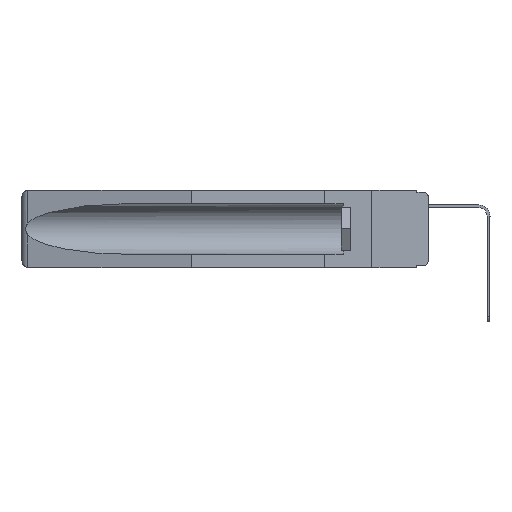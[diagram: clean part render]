
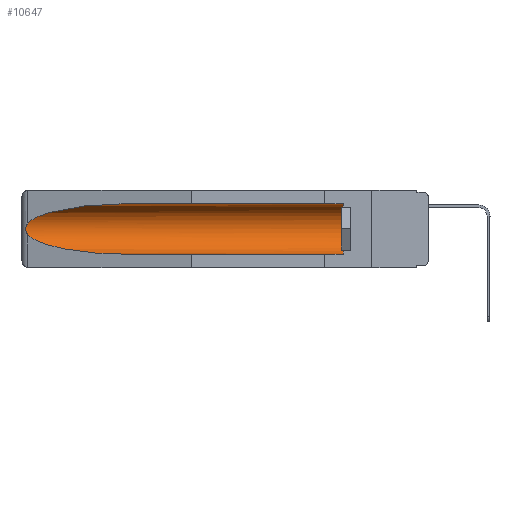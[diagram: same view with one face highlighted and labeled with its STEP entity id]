
A CAD part, left-side view. The second image highlights one B-rep face of the part: STEP entity #10647.
In plain terms, the highlighted cylindrical face has radius 2.857 mm (diameter 5.715 mm), a partial arc.
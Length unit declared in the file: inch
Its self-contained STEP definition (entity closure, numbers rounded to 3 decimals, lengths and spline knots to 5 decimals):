
#420 = ORIENTED_EDGE ( 'NONE', *, *, #8648, .T. ) ;
#556 = CARTESIAN_POINT ( 'NONE',  ( 0.26537, 1.52718, -0.14972 ) ) ;
#618 = CARTESIAN_POINT ( 'NONE',  ( 0.155, 0.126, -0.284 ) ) ;
#1418 = CARTESIAN_POINT ( 'NONE',  ( 0.2673, 1.53269, -0.17917 ) ) ;
#1465 = CARTESIAN_POINT ( 'NONE',  ( 0.26537, 1.52718, -0.14972 ) ) ;
#1823 = DIRECTION ( 'NONE',  ( 0., 1., 0. ) ) ;
#1854 = CYLINDRICAL_SURFACE ( 'NONE', #3262, 0.1125 ) ;
#1865 = VERTEX_POINT ( 'NONE', #3945 ) ;
#1936 = CARTESIAN_POINT ( 'NONE',  ( 0.155, -0.30754, -0.059 ) ) ;
#2005 = VECTOR ( 'NONE', #16226, 39.37008 ) ;
#2020 = CARTESIAN_POINT ( 'NONE',  ( 0.26537, 1.52718, -0.14972 ) ) ;
#2092 = CARTESIAN_POINT ( 'NONE',  ( 0.155, -0.30754, -0.284 ) ) ;
#2110 = CARTESIAN_POINT ( 'NONE',  ( 0.26537, 1.52718, -0.19328 ) ) ;
#2526 = CARTESIAN_POINT ( 'NONE',  ( 0.26597, 1.52961, -0.15275 ) ) ;
#2699 = EDGE_CURVE ( 'NONE', #8354, #8867, #6921, .T. ) ;
#2708 = LINE ( 'NONE', #1936, #8896 ) ;
#2745 = CARTESIAN_POINT ( 'NONE',  ( 0.2675, 1.53308, -0.16763 ) ) ;
#2892 = EDGE_CURVE ( 'NONE', #11684, #8867, #15221, .T. ) ;
#3136 = ORIENTED_EDGE ( 'NONE', *, *, #15280, .T. ) ;
#3262 = AXIS2_PLACEMENT_3D ( 'NONE', #7051, #12228, #11051 ) ;
#3314 = CARTESIAN_POINT ( 'NONE',  ( 0.155, 0.126, -0.1715 ) ) ;
#3534 = ORIENTED_EDGE ( 'NONE', *, *, #5047, .T. ) ;
#3752 = VERTEX_POINT ( 'NONE', #2020 ) ;
#3945 = CARTESIAN_POINT ( 'NONE',  ( 0.155, 0.126, -0.059 ) ) ;
#4772 = CARTESIAN_POINT ( 'NONE',  ( 0.21114, 1.30732, -0.284 ) ) ;
#5047 = EDGE_CURVE ( 'NONE', #11684, #1865, #5477, .T. ) ;
#5470 = CARTESIAN_POINT ( 'NONE',  ( 0.155, 1.07973, -0.059 ) ) ;
#5477 = CIRCLE ( 'NONE', #8446, 0.1125 ) ;
#5877 = CARTESIAN_POINT ( 'NONE',  ( 0.155, 1.07973, -0.284 ) ) ;
#6402 = CARTESIAN_POINT ( 'NONE',  ( 0.26537, 1.52718, -0.19328 ) ) ;
#6573 = CARTESIAN_POINT ( 'NONE',  ( 0.2675, 1.53308, -0.17534 ) ) ;
#6921 =( BOUNDED_CURVE ( )  B_SPLINE_CURVE ( 3, ( #2110, #11060, #4772, #14901 ),
 .UNSPECIFIED., .F., .F. ) 
 B_SPLINE_CURVE_WITH_KNOTS ( ( 4, 4 ),
 ( 0.1948, 1.5708 ),
 .UNSPECIFIED. ) 
 CURVE ( )  GEOMETRIC_REPRESENTATION_ITEM ( )  RATIONAL_B_SPLINE_CURVE ( ( 1., 0.848, 0.848, 1. ) ) 
 REPRESENTATION_ITEM ( '' )  );
#7051 = CARTESIAN_POINT ( 'NONE',  ( 0.155, -0.30754, -0.1715 ) ) ;
#7501 = EDGE_CURVE ( 'NONE', #15870, #3752, #10529, .T. ) ;
#7812 = CARTESIAN_POINT ( 'NONE',  ( 0.26655, 1.53094, -0.18657 ) ) ;
#8151 = CARTESIAN_POINT ( 'NONE',  ( 0.25451, 1.48313, -0.09465 ) ) ;
#8354 = VERTEX_POINT ( 'NONE', #13441 ) ;
#8446 = AXIS2_PLACEMENT_3D ( 'NONE', #3314, #13560, #10818 ) ;
#8648 = EDGE_CURVE ( 'NONE', #1865, #15870, #2708, .T. ) ;
#8867 = VERTEX_POINT ( 'NONE', #5877 ) ;
#8896 = VECTOR ( 'NONE', #1823, 39.37008 ) ;
#9047 = CARTESIAN_POINT ( 'NONE',  ( 0.26654, 1.53092, -0.15636 ) ) ;
#9292 = B_SPLINE_CURVE_WITH_KNOTS ( 'NONE', 3,
 ( #1465, #2526, #9047, #12829, #2745, #6573, #1418, #7812, #11484, #6402 ),
 .UNSPECIFIED., .F., .F.,
 ( 4, 2, 2, 2, 4 ),
 ( 0., 0.00029, 0.00058, 0.00087, 0.00117 ),
 .UNSPECIFIED. ) ;
#10529 =( BOUNDED_CURVE ( )  B_SPLINE_CURVE ( 3, ( #5470, #14427, #8151, #556 ),
 .UNSPECIFIED., .F., .F. ) 
 B_SPLINE_CURVE_WITH_KNOTS ( ( 4, 4 ),
 ( 4.71239, 6.08839 ),
 .UNSPECIFIED. ) 
 CURVE ( )  GEOMETRIC_REPRESENTATION_ITEM ( )  RATIONAL_B_SPLINE_CURVE ( ( 1., 0.848, 0.848, 1. ) ) 
 REPRESENTATION_ITEM ( '' )  );
#10647 = ADVANCED_FACE ( 'NONE', ( #14852 ), #1854, .F. ) ;
#10678 = ORIENTED_EDGE ( 'NONE', *, *, #7501, .T. ) ;
#10818 = DIRECTION ( 'NONE',  ( 0., 0., 1. ) ) ;
#11051 = DIRECTION ( 'NONE',  ( 0., 0., 1. ) ) ;
#11060 = CARTESIAN_POINT ( 'NONE',  ( 0.25451, 1.48313, -0.24835 ) ) ;
#11484 = CARTESIAN_POINT ( 'NONE',  ( 0.26597, 1.5296, -0.19026 ) ) ;
#11684 = VERTEX_POINT ( 'NONE', #618 ) ;
#12228 = DIRECTION ( 'NONE',  ( 0., 1., 0. ) ) ;
#12829 = CARTESIAN_POINT ( 'NONE',  ( 0.2673, 1.5327, -0.16383 ) ) ;
#13441 = CARTESIAN_POINT ( 'NONE',  ( 0.26537, 1.52718, -0.19328 ) ) ;
#13560 = DIRECTION ( 'NONE',  ( 0., -1., 0. ) ) ;
#14427 = CARTESIAN_POINT ( 'NONE',  ( 0.21114, 1.30732, -0.059 ) ) ;
#14721 = EDGE_LOOP ( 'NONE', ( #10678, #3136, #16037, #15196, #3534, #420 ) ) ;
#14852 = FACE_OUTER_BOUND ( 'NONE', #14721, .T. ) ;
#14901 = CARTESIAN_POINT ( 'NONE',  ( 0.155, 1.07973, -0.284 ) ) ;
#15196 = ORIENTED_EDGE ( 'NONE', *, *, #2892, .F. ) ;
#15221 = LINE ( 'NONE', #2092, #2005 ) ;
#15280 = EDGE_CURVE ( 'NONE', #3752, #8354, #9292, .T. ) ;
#15382 = CARTESIAN_POINT ( 'NONE',  ( 0.155, 1.07973, -0.059 ) ) ;
#15870 = VERTEX_POINT ( 'NONE', #15382 ) ;
#16037 = ORIENTED_EDGE ( 'NONE', *, *, #2699, .T. ) ;
#16226 = DIRECTION ( 'NONE',  ( 0., 1., 0. ) ) ;
